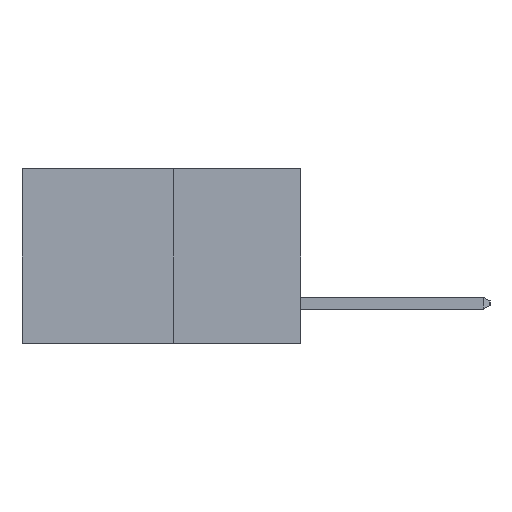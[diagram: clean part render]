
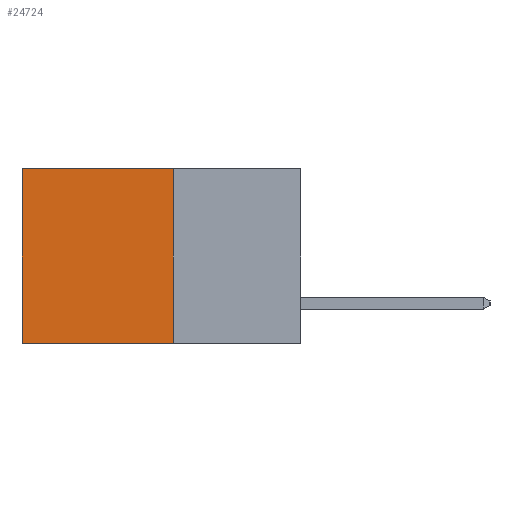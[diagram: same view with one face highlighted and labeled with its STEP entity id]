
A CAD part, left-side view. The second image highlights one B-rep face of the part: STEP entity #24724.
In plain terms, the highlighted planar face has unit normal (-1, 0, 0).
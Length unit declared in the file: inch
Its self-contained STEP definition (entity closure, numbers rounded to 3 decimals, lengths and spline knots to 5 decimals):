
#1119 = DIRECTION ( 'NONE',  ( 0., 0., -1. ) ) ;
#1959 = LINE ( 'NONE', #20434, #21752 ) ;
#2512 = VECTOR ( 'NONE', #16321, 39.37008 ) ;
#2781 = CARTESIAN_POINT ( 'NONE',  ( 0.277, 0.59, 0. ) ) ;
#2849 = CARTESIAN_POINT ( 'NONE',  ( 0.277, 0.59, -0.37 ) ) ;
#3301 = AXIS2_PLACEMENT_3D ( 'NONE', #23998, #12686, #1119 ) ;
#3866 = ORIENTED_EDGE ( 'NONE', *, *, #7720, .T. ) ;
#3984 = VERTEX_POINT ( 'NONE', #10252 ) ;
#5193 = LINE ( 'NONE', #20816, #19871 ) ;
#5829 = VERTEX_POINT ( 'NONE', #2781 ) ;
#6734 = ORIENTED_EDGE ( 'NONE', *, *, #21637, .F. ) ;
#7109 = CARTESIAN_POINT ( 'NONE',  ( 0.277, 0.27, -0.37 ) ) ;
#7161 = DIRECTION ( 'NONE',  ( 0., 1., 0. ) ) ;
#7720 = EDGE_CURVE ( 'NONE', #9400, #5829, #1959, .T. ) ;
#8420 = ORIENTED_EDGE ( 'NONE', *, *, #9519, .F. ) ;
#8746 = CARTESIAN_POINT ( 'NONE',  ( 0.277, 0.27, 0. ) ) ;
#8894 = LINE ( 'NONE', #2849, #2512 ) ;
#9028 = DIRECTION ( 'NONE',  ( 0., 0., -1. ) ) ;
#9070 = VECTOR ( 'NONE', #9028, 39.37008 ) ;
#9400 = VERTEX_POINT ( 'NONE', #8746 ) ;
#9519 = EDGE_CURVE ( 'NONE', #11656, #3984, #5193, .T. ) ;
#10252 = CARTESIAN_POINT ( 'NONE',  ( 0.277, 0.59, -0.37 ) ) ;
#10824 = PLANE ( 'NONE',  #3301 ) ;
#11157 = EDGE_LOOP ( 'NONE', ( #21111, #8420, #6734, #3866 ) ) ;
#11656 = VERTEX_POINT ( 'NONE', #16843 ) ;
#12686 = DIRECTION ( 'NONE',  ( 1., 0., 0. ) ) ;
#16321 = DIRECTION ( 'NONE',  ( 0., 0., -1. ) ) ;
#16843 = CARTESIAN_POINT ( 'NONE',  ( 0.277, 0.27, -0.37 ) ) ;
#18758 = EDGE_CURVE ( 'NONE', #5829, #3984, #8894, .T. ) ;
#19871 = VECTOR ( 'NONE', #7161, 39.37008 ) ;
#20429 = DIRECTION ( 'NONE',  ( 0., 1., 0. ) ) ;
#20434 = CARTESIAN_POINT ( 'NONE',  ( 0.277, 0.27, 0. ) ) ;
#20816 = CARTESIAN_POINT ( 'NONE',  ( 0.277, 0.27, -0.37 ) ) ;
#21111 = ORIENTED_EDGE ( 'NONE', *, *, #18758, .T. ) ;
#21637 = EDGE_CURVE ( 'NONE', #9400, #11656, #24161, .T. ) ;
#21752 = VECTOR ( 'NONE', #20429, 39.37008 ) ;
#23388 = FACE_OUTER_BOUND ( 'NONE', #11157, .T. ) ;
#23998 = CARTESIAN_POINT ( 'NONE',  ( 0.277, 0.27, -0.37 ) ) ;
#24161 = LINE ( 'NONE', #7109, #9070 ) ;
#24724 = ADVANCED_FACE ( 'NONE', ( #23388 ), #10824, .F. ) ;
